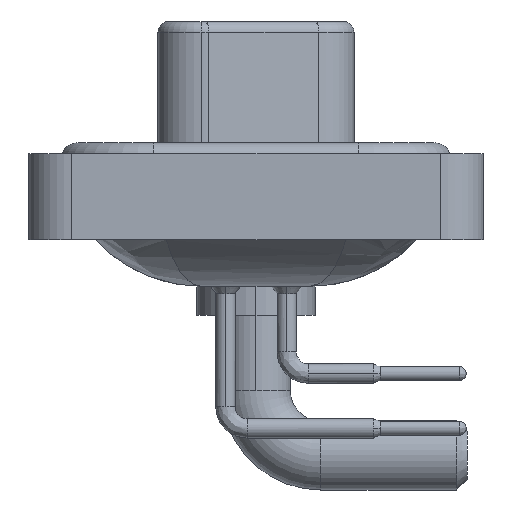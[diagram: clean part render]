
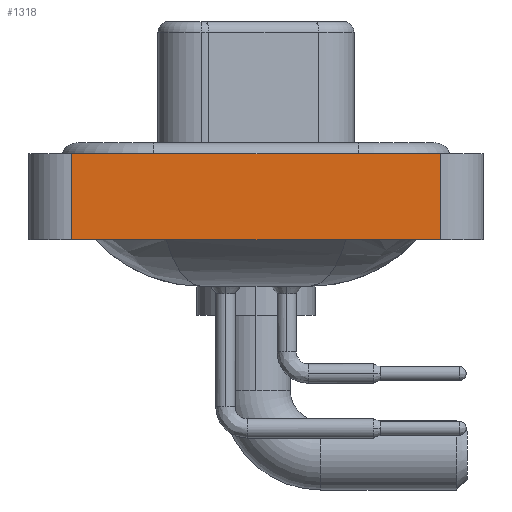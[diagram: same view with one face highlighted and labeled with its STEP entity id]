
A CAD part, left-side view. The second image highlights one B-rep face of the part: STEP entity #1318.
In plain terms, the highlighted planar face has unit normal (-1, 0, 0).
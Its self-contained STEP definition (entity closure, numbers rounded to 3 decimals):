
#120 = ORIENTED_EDGE ( 'NONE', *, *, #13990, .T. ) ;
#360 = VECTOR ( 'NONE', #10251, 1000. ) ;
#1197 = VERTEX_POINT ( 'NONE', #15682 ) ;
#1278 = CARTESIAN_POINT ( 'NONE',  ( -7.35, -8.55, -3.6 ) ) ;
#1318 = ADVANCED_FACE ( 'NONE', ( #9535 ), #4444, .T. ) ;
#2200 = DIRECTION ( 'NONE',  ( -1., 0., 0. ) ) ;
#2833 = DIRECTION ( 'NONE',  ( 0., -1., 0. ) ) ;
#3595 = LINE ( 'NONE', #24220, #27790 ) ;
#3740 = DIRECTION ( 'NONE',  ( 0., 0., 1. ) ) ;
#4072 = VECTOR ( 'NONE', #5896, 1000. ) ;
#4444 = PLANE ( 'NONE',  #5905 ) ;
#5896 = DIRECTION ( 'NONE',  ( 0., 0., 1. ) ) ;
#5905 = AXIS2_PLACEMENT_3D ( 'NONE', #11171, #2200, #18660 ) ;
#8466 = ORIENTED_EDGE ( 'NONE', *, *, #11860, .T. ) ;
#9535 = FACE_OUTER_BOUND ( 'NONE', #16449, .T. ) ;
#9919 = ORIENTED_EDGE ( 'NONE', *, *, #16576, .F. ) ;
#10251 = DIRECTION ( 'NONE',  ( 0., -1., 0. ) ) ;
#11171 = CARTESIAN_POINT ( 'NONE',  ( -7.35, -8.55, -3.6 ) ) ;
#11860 = EDGE_CURVE ( 'NONE', #16815, #1197, #20104, .T. ) ;
#13132 = VERTEX_POINT ( 'NONE', #14429 ) ;
#13990 = EDGE_CURVE ( 'NONE', #14962, #16815, #23311, .T. ) ;
#14429 = CARTESIAN_POINT ( 'NONE',  ( -7.35, 8.55, 0.4 ) ) ;
#14962 = VERTEX_POINT ( 'NONE', #18875 ) ;
#15327 = CARTESIAN_POINT ( 'NONE',  ( -7.35, -8.55, -3.6 ) ) ;
#15682 = CARTESIAN_POINT ( 'NONE',  ( -7.35, -8.55, 0.4 ) ) ;
#16449 = EDGE_LOOP ( 'NONE', ( #8466, #27396, #9919, #120 ) ) ;
#16452 = CARTESIAN_POINT ( 'NONE',  ( -7.35, -8.55, -3.6 ) ) ;
#16576 = EDGE_CURVE ( 'NONE', #14962, #13132, #3595, .T. ) ;
#16815 = VERTEX_POINT ( 'NONE', #1278 ) ;
#18660 = DIRECTION ( 'NONE',  ( 0., 0., 1. ) ) ;
#18875 = CARTESIAN_POINT ( 'NONE',  ( -7.35, 8.55, -3.6 ) ) ;
#19077 = VECTOR ( 'NONE', #2833, 1000. ) ;
#19384 = CARTESIAN_POINT ( 'NONE',  ( -7.35, -8.55, 0.4 ) ) ;
#20104 = LINE ( 'NONE', #15327, #4072 ) ;
#20238 = EDGE_CURVE ( 'NONE', #13132, #1197, #28933, .T. ) ;
#23311 = LINE ( 'NONE', #16452, #19077 ) ;
#24220 = CARTESIAN_POINT ( 'NONE',  ( -7.35, 8.55, -3.6 ) ) ;
#27396 = ORIENTED_EDGE ( 'NONE', *, *, #20238, .F. ) ;
#27790 = VECTOR ( 'NONE', #3740, 1000. ) ;
#28933 = LINE ( 'NONE', #19384, #360 ) ;
